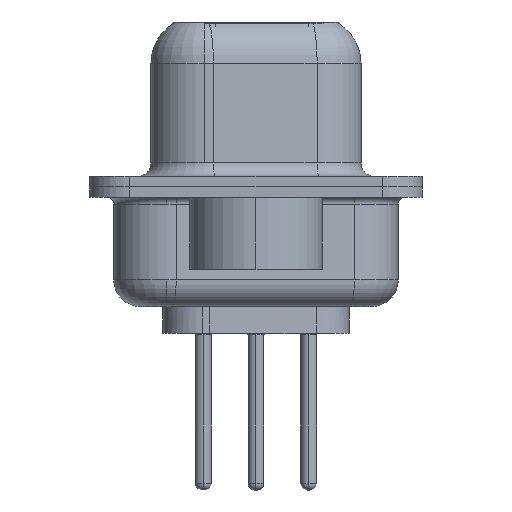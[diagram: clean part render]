
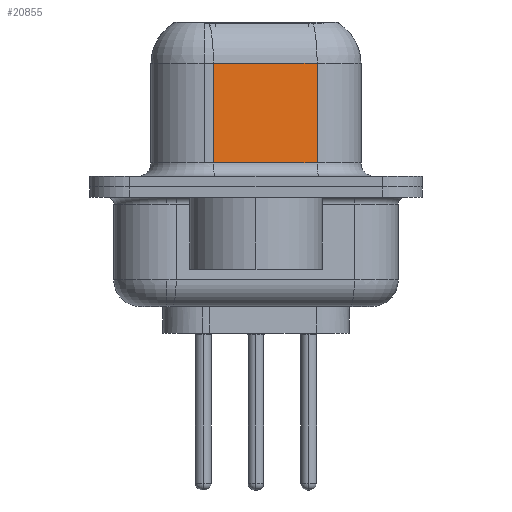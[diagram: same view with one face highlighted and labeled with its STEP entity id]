
A CAD part, left-side view. The second image highlights one B-rep face of the part: STEP entity #20855.
In plain terms, the highlighted planar face has unit normal (-0.985, -0.174, 0).
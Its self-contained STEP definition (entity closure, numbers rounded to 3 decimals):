
#458 = CARTESIAN_POINT ( 'NONE',  ( 5.068, -2.297, 0.9 ) ) ;
#997 = CARTESIAN_POINT ( 'NONE',  ( 4.38, 1.603, 6.4 ) ) ;
#1029 = FACE_OUTER_BOUND ( 'NONE', #9735, .T. ) ;
#1236 = ORIENTED_EDGE ( 'NONE', *, *, #12840, .F. ) ;
#1887 = VERTEX_POINT ( 'NONE', #12017 ) ;
#3429 = DIRECTION ( 'NONE',  ( -0.174, 0.985, 0. ) ) ;
#3813 = EDGE_CURVE ( 'NONE', #10903, #1887, #14246, .T. ) ;
#4722 = CARTESIAN_POINT ( 'NONE',  ( 5.068, -2.297, 0.9 ) ) ;
#5231 = AXIS2_PLACEMENT_3D ( 'NONE', #22767, #15873, #23474 ) ;
#5361 = ORIENTED_EDGE ( 'NONE', *, *, #17696, .T. ) ;
#6176 = VERTEX_POINT ( 'NONE', #6807 ) ;
#6566 = LINE ( 'NONE', #997, #7177 ) ;
#6807 = CARTESIAN_POINT ( 'NONE',  ( 4.38, 1.603, 0.9 ) ) ;
#7177 = VECTOR ( 'NONE', #10130, 1000. ) ;
#7367 = CARTESIAN_POINT ( 'NONE',  ( 5.068, -2.297, 4.65 ) ) ;
#8260 = PLANE ( 'NONE',  #5231 ) ;
#9735 = EDGE_LOOP ( 'NONE', ( #1236, #14449, #12638, #5361 ) ) ;
#10130 = DIRECTION ( 'NONE',  ( 0., 0., -1. ) ) ;
#10903 = VERTEX_POINT ( 'NONE', #7367 ) ;
#12017 = CARTESIAN_POINT ( 'NONE',  ( 4.38, 1.603, 4.65 ) ) ;
#12638 = ORIENTED_EDGE ( 'NONE', *, *, #14080, .T. ) ;
#12840 = EDGE_CURVE ( 'NONE', #10903, #14465, #17597, .T. ) ;
#13414 = DIRECTION ( 'NONE',  ( 0.174, -0.985, 0. ) ) ;
#14080 = EDGE_CURVE ( 'NONE', #1887, #6176, #6566, .T. ) ;
#14246 = LINE ( 'NONE', #21258, #16761 ) ;
#14449 = ORIENTED_EDGE ( 'NONE', *, *, #3813, .T. ) ;
#14465 = VERTEX_POINT ( 'NONE', #4722 ) ;
#15187 = LINE ( 'NONE', #458, #19289 ) ;
#15873 = DIRECTION ( 'NONE',  ( 0.985, 0.174, 0. ) ) ;
#16761 = VECTOR ( 'NONE', #3429, 1000. ) ;
#17597 = LINE ( 'NONE', #20926, #19199 ) ;
#17696 = EDGE_CURVE ( 'NONE', #6176, #14465, #15187, .T. ) ;
#19199 = VECTOR ( 'NONE', #19266, 1000. ) ;
#19266 = DIRECTION ( 'NONE',  ( 0., 0., -1. ) ) ;
#19289 = VECTOR ( 'NONE', #13414, 1000. ) ;
#20855 = ADVANCED_FACE ( 'NONE', ( #1029 ), #8260, .F. ) ;
#20926 = CARTESIAN_POINT ( 'NONE',  ( 5.068, -2.297, 6.4 ) ) ;
#21258 = CARTESIAN_POINT ( 'NONE',  ( 5.068, -2.297, 4.65 ) ) ;
#22767 = CARTESIAN_POINT ( 'NONE',  ( 5.068, -2.297, 6.4 ) ) ;
#23474 = DIRECTION ( 'NONE',  ( -0.174, 0.985, 0. ) ) ;
